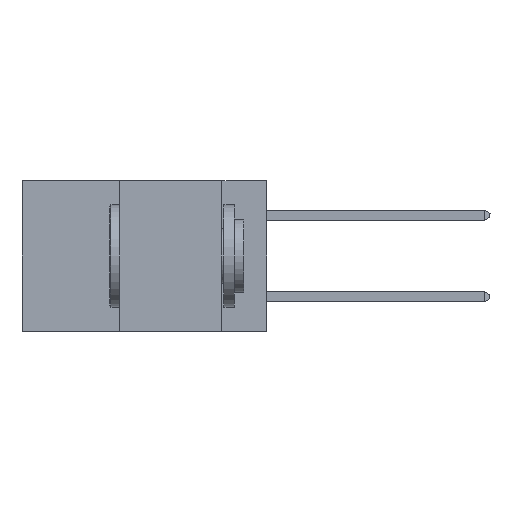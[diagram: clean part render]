
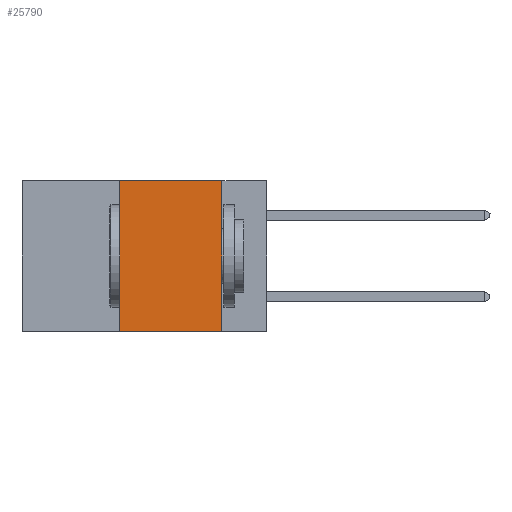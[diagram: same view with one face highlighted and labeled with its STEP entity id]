
A CAD part, left-side view. The second image highlights one B-rep face of the part: STEP entity #25790.
In plain terms, the highlighted planar face has unit normal (-1, 0, 0).
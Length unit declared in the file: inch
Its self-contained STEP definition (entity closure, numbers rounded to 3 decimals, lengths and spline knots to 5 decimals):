
#540 = VECTOR ( 'NONE', #19367, 39.37008 ) ;
#2038 = CARTESIAN_POINT ( 'NONE',  ( 0., 0.11, 0. ) ) ;
#2560 = EDGE_CURVE ( 'NONE', #25923, #18141, #3824, .T. ) ;
#2847 = VERTEX_POINT ( 'NONE', #2038 ) ;
#3824 = LINE ( 'NONE', #16544, #44011 ) ;
#8818 = PLANE ( 'NONE',  #31610 ) ;
#9007 = LINE ( 'NONE', #16087, #21147 ) ;
#9187 = DIRECTION ( 'NONE',  ( 0., -1., 0. ) ) ;
#11129 = ORIENTED_EDGE ( 'NONE', *, *, #38361, .T. ) ;
#11799 = VERTEX_POINT ( 'NONE', #30018 ) ;
#12594 = LINE ( 'NONE', #22792, #35708 ) ;
#14334 = EDGE_CURVE ( 'NONE', #2847, #11799, #9007, .T. ) ;
#15076 = EDGE_LOOP ( 'NONE', ( #20160, #41248, #23810, #11129 ) ) ;
#16087 = CARTESIAN_POINT ( 'NONE',  ( 0., 0.11, 0. ) ) ;
#16544 = CARTESIAN_POINT ( 'NONE',  ( 0., 0.36, 0. ) ) ;
#18141 = VERTEX_POINT ( 'NONE', #21745 ) ;
#19367 = DIRECTION ( 'NONE',  ( 0., -1., 0. ) ) ;
#19611 = DIRECTION ( 'NONE',  ( 1., 0., 0. ) ) ;
#19918 = FACE_OUTER_BOUND ( 'NONE', #15076, .T. ) ;
#20100 = DIRECTION ( 'NONE',  ( 0., 0., 1. ) ) ;
#20160 = ORIENTED_EDGE ( 'NONE', *, *, #14334, .F. ) ;
#21147 = VECTOR ( 'NONE', #40770, 39.37008 ) ;
#21482 = LINE ( 'NONE', #44051, #540 ) ;
#21745 = CARTESIAN_POINT ( 'NONE',  ( 0., 0.36, 0. ) ) ;
#22792 = CARTESIAN_POINT ( 'NONE',  ( 0., 0.6, -0.37 ) ) ;
#23810 = ORIENTED_EDGE ( 'NONE', *, *, #2560, .F. ) ;
#25790 = ADVANCED_FACE ( 'NONE', ( #19918 ), #8818, .F. ) ;
#25923 = VERTEX_POINT ( 'NONE', #41223 ) ;
#26952 = EDGE_CURVE ( 'NONE', #18141, #2847, #21482, .T. ) ;
#30018 = CARTESIAN_POINT ( 'NONE',  ( 0., 0.11, -0.37 ) ) ;
#30034 = DIRECTION ( 'NONE',  ( 0., 0., -1. ) ) ;
#31610 = AXIS2_PLACEMENT_3D ( 'NONE', #33418, #19611, #30034 ) ;
#33418 = CARTESIAN_POINT ( 'NONE',  ( 0., 0.6, 0. ) ) ;
#35708 = VECTOR ( 'NONE', #9187, 39.37008 ) ;
#38361 = EDGE_CURVE ( 'NONE', #25923, #11799, #12594, .T. ) ;
#40770 = DIRECTION ( 'NONE',  ( 0., 0., -1. ) ) ;
#41223 = CARTESIAN_POINT ( 'NONE',  ( 0., 0.36, -0.37 ) ) ;
#41248 = ORIENTED_EDGE ( 'NONE', *, *, #26952, .F. ) ;
#44011 = VECTOR ( 'NONE', #20100, 39.37008 ) ;
#44051 = CARTESIAN_POINT ( 'NONE',  ( 0., 0.6, 0. ) ) ;
